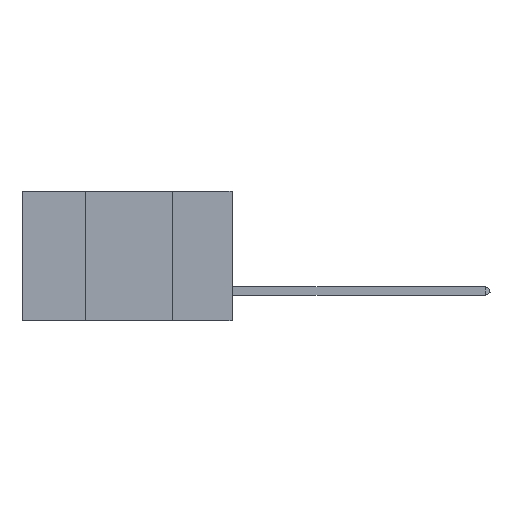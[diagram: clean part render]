
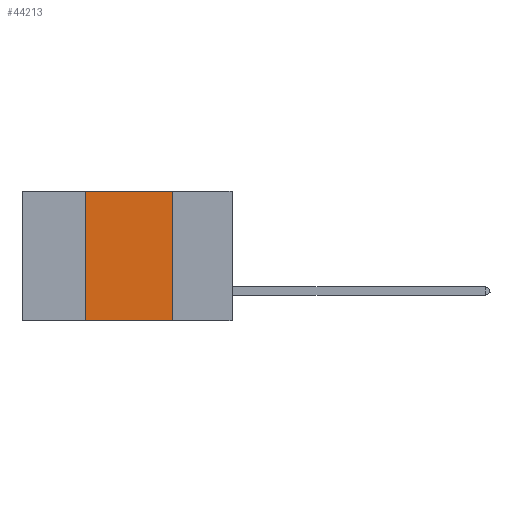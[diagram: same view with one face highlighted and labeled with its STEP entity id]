
A CAD part, left-side view. The second image highlights one B-rep face of the part: STEP entity #44213.
In plain terms, the highlighted planar face has unit normal (-1, 0, 0).
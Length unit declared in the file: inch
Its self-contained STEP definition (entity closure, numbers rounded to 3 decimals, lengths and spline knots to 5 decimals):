
#2290 = CARTESIAN_POINT ( 'NONE',  ( 0., 0.6, -0.37 ) ) ;
#6284 = DIRECTION ( 'NONE',  ( 0., 0., -1. ) ) ;
#6966 = EDGE_LOOP ( 'NONE', ( #15731, #44897, #8078, #44866 ) ) ;
#7649 = EDGE_CURVE ( 'NONE', #40221, #15424, #9615, .T. ) ;
#8078 = ORIENTED_EDGE ( 'NONE', *, *, #29974, .F. ) ;
#9615 = LINE ( 'NONE', #13168, #23196 ) ;
#9633 = DIRECTION ( 'NONE',  ( 0., -1., 0. ) ) ;
#10579 = VECTOR ( 'NONE', #34314, 39.37008 ) ;
#11830 = CARTESIAN_POINT ( 'NONE',  ( 0., 0.42, 0. ) ) ;
#13168 = CARTESIAN_POINT ( 'NONE',  ( 0., 0.17, 0. ) ) ;
#15354 = DIRECTION ( 'NONE',  ( 1., 0., 0. ) ) ;
#15424 = VERTEX_POINT ( 'NONE', #16208 ) ;
#15731 = ORIENTED_EDGE ( 'NONE', *, *, #7649, .F. ) ;
#15940 = EDGE_CURVE ( 'NONE', #29630, #15424, #20339, .T. ) ;
#15995 = PLANE ( 'NONE',  #29226 ) ;
#16208 = CARTESIAN_POINT ( 'NONE',  ( 0., 0.17, -0.37 ) ) ;
#20339 = LINE ( 'NONE', #2290, #41311 ) ;
#23196 = VECTOR ( 'NONE', #6284, 39.37008 ) ;
#26034 = EDGE_CURVE ( 'NONE', #28416, #40221, #29238, .T. ) ;
#28416 = VERTEX_POINT ( 'NONE', #31074 ) ;
#29226 = AXIS2_PLACEMENT_3D ( 'NONE', #33512, #15354, #40733 ) ;
#29238 = LINE ( 'NONE', #30299, #10579 ) ;
#29630 = VERTEX_POINT ( 'NONE', #45505 ) ;
#29974 = EDGE_CURVE ( 'NONE', #29630, #28416, #46618, .T. ) ;
#30299 = CARTESIAN_POINT ( 'NONE',  ( 0., 0.6, 0. ) ) ;
#31074 = CARTESIAN_POINT ( 'NONE',  ( 0., 0.42, 0. ) ) ;
#32415 = FACE_OUTER_BOUND ( 'NONE', #6966, .T. ) ;
#33512 = CARTESIAN_POINT ( 'NONE',  ( 0., 0.6, 0. ) ) ;
#33696 = CARTESIAN_POINT ( 'NONE',  ( 0., 0.17, 0. ) ) ;
#34314 = DIRECTION ( 'NONE',  ( 0., -1., 0. ) ) ;
#40221 = VERTEX_POINT ( 'NONE', #33696 ) ;
#40733 = DIRECTION ( 'NONE',  ( 0., 0., -1. ) ) ;
#41311 = VECTOR ( 'NONE', #9633, 39.37008 ) ;
#44213 = ADVANCED_FACE ( 'NONE', ( #32415 ), #15995, .F. ) ;
#44866 = ORIENTED_EDGE ( 'NONE', *, *, #15940, .T. ) ;
#44897 = ORIENTED_EDGE ( 'NONE', *, *, #26034, .F. ) ;
#45433 = DIRECTION ( 'NONE',  ( 0., 0., 1. ) ) ;
#45505 = CARTESIAN_POINT ( 'NONE',  ( 0., 0.42, -0.37 ) ) ;
#46161 = VECTOR ( 'NONE', #45433, 39.37008 ) ;
#46618 = LINE ( 'NONE', #11830, #46161 ) ;
